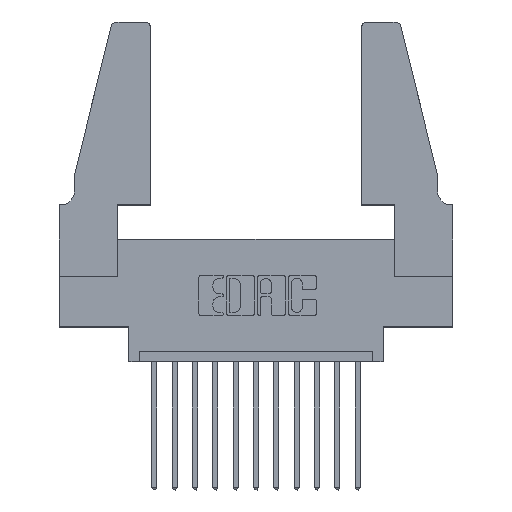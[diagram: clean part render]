
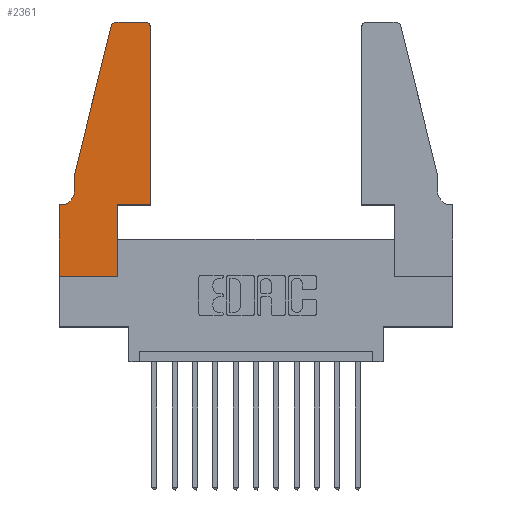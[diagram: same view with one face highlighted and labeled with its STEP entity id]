
A CAD part, top view. The second image highlights one B-rep face of the part: STEP entity #2361.
In plain terms, the highlighted planar face has unit normal (0, 0, 1).
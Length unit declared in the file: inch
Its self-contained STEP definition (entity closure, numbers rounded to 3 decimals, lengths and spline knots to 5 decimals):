
#89 = CARTESIAN_POINT ( 'NONE',  ( 0.4505, 0.35, 0.37 ) ) ;
#116 = CARTESIAN_POINT ( 'NONE',  ( 0.25487, 1.22718, 0.37 ) ) ;
#725 = CARTESIAN_POINT ( 'NONE',  ( 0.4505, 0.35, 0.37 ) ) ;
#737 = EDGE_CURVE ( 'NONE', #4386, #1891, #3913, .T. ) ;
#766 = LINE ( 'NONE', #13095, #12491 ) ;
#920 = EDGE_CURVE ( 'NONE', #3782, #13188, #6446, .T. ) ;
#1438 = DIRECTION ( 'NONE',  ( 0., 0., 1. ) ) ;
#1468 = DIRECTION ( 'NONE',  ( 1., 0., 0. ) ) ;
#1543 = VECTOR ( 'NONE', #6081, 39.37008 ) ;
#1684 = DIRECTION ( 'NONE',  ( 0., -1., 0. ) ) ;
#1845 = EDGE_CURVE ( 'NONE', #1891, #2045, #13556, .T. ) ;
#1891 = VERTEX_POINT ( 'NONE', #8064 ) ;
#2045 = VERTEX_POINT ( 'NONE', #2785 ) ;
#2224 = LINE ( 'NONE', #14185, #1543 ) ;
#2236 = VERTEX_POINT ( 'NONE', #14622 ) ;
#2361 = ADVANCED_FACE ( 'NONE', ( #10120 ), #10490, .T. ) ;
#2376 = EDGE_CURVE ( 'NONE', #3170, #7698, #11215, .T. ) ;
#2407 = ORIENTED_EDGE ( 'NONE', *, *, #13330, .T. ) ;
#2785 = CARTESIAN_POINT ( 'NONE',  ( 0., 0.35, 0.37 ) ) ;
#2909 = DIRECTION ( 'NONE',  ( 0., 1., 0. ) ) ;
#2993 = LINE ( 'NONE', #14517, #6554 ) ;
#3170 = VERTEX_POINT ( 'NONE', #116 ) ;
#3244 = LINE ( 'NONE', #6177, #12352 ) ;
#3681 = DIRECTION ( 'NONE',  ( 1., 0., 0. ) ) ;
#3738 = ORIENTED_EDGE ( 'NONE', *, *, #2376, .T. ) ;
#3782 = VERTEX_POINT ( 'NONE', #89 ) ;
#3790 = CARTESIAN_POINT ( 'NONE',  ( 0.0755, 0.5, 0.37 ) ) ;
#3913 = CIRCLE ( 'NONE', #10868, 0.07 ) ;
#4011 = CARTESIAN_POINT ( 'NONE',  ( 0.2865, 0.35, 0.37 ) ) ;
#4113 = ORIENTED_EDGE ( 'NONE', *, *, #9450, .T. ) ;
#4261 = DIRECTION ( 'NONE',  ( 0., 1., 0. ) ) ;
#4386 = VERTEX_POINT ( 'NONE', #6776 ) ;
#4493 = CARTESIAN_POINT ( 'NONE',  ( 0.0055, 0.42, 0.37 ) ) ;
#4815 = DIRECTION ( 'NONE',  ( -0.239, -0.971, 0. ) ) ;
#4913 = CIRCLE ( 'NONE', #4923, 0.03 ) ;
#4922 = DIRECTION ( 'NONE',  ( 0., 0., 1. ) ) ;
#4923 = AXIS2_PLACEMENT_3D ( 'NONE', #12338, #12143, #13402 ) ;
#4983 = VECTOR ( 'NONE', #12726, 39.37008 ) ;
#5013 = CARTESIAN_POINT ( 'NONE',  ( 0.0755, 0.5, 0.37 ) ) ;
#5110 = ORIENTED_EDGE ( 'NONE', *, *, #11176, .T. ) ;
#5371 = VERTEX_POINT ( 'NONE', #7782 ) ;
#5526 = AXIS2_PLACEMENT_3D ( 'NONE', #9406, #4922, #1468 ) ;
#5924 = ORIENTED_EDGE ( 'NONE', *, *, #8864, .T. ) ;
#6081 = DIRECTION ( 'NONE',  ( 1., 0., 0. ) ) ;
#6177 = CARTESIAN_POINT ( 'NONE',  ( 0.2605, 1.25, 0.37 ) ) ;
#6446 = LINE ( 'NONE', #725, #7123 ) ;
#6554 = VECTOR ( 'NONE', #4261, 39.37008 ) ;
#6776 = CARTESIAN_POINT ( 'NONE',  ( 0.0755, 0.42, 0.37 ) ) ;
#7045 = VERTEX_POINT ( 'NONE', #13033 ) ;
#7113 = LINE ( 'NONE', #11530, #4983 ) ;
#7123 = VECTOR ( 'NONE', #2909, 39.37008 ) ;
#7177 = VECTOR ( 'NONE', #11707, 39.37008 ) ;
#7354 = EDGE_CURVE ( 'NONE', #14381, #14234, #2993, .T. ) ;
#7688 = CIRCLE ( 'NONE', #11392, 0.03 ) ;
#7698 = VERTEX_POINT ( 'NONE', #3790 ) ;
#7782 = CARTESIAN_POINT ( 'NONE',  ( 0., 0., 0.37 ) ) ;
#8064 = CARTESIAN_POINT ( 'NONE',  ( 0.0055, 0.35, 0.37 ) ) ;
#8535 = VECTOR ( 'NONE', #9864, 39.37008 ) ;
#8864 = EDGE_CURVE ( 'NONE', #7698, #4386, #12046, .T. ) ;
#8868 = ORIENTED_EDGE ( 'NONE', *, *, #737, .T. ) ;
#8895 = ORIENTED_EDGE ( 'NONE', *, *, #7354, .T. ) ;
#9120 = DIRECTION ( 'NONE',  ( -1., 0., 0. ) ) ;
#9406 = CARTESIAN_POINT ( 'NONE',  ( 0., 0.35, 0.37 ) ) ;
#9450 = EDGE_CURVE ( 'NONE', #7045, #3170, #7688, .T. ) ;
#9759 = DIRECTION ( 'NONE',  ( -1., 0., 0. ) ) ;
#9864 = DIRECTION ( 'NONE',  ( -1., 0., 0. ) ) ;
#10120 = FACE_OUTER_BOUND ( 'NONE', #14323, .T. ) ;
#10127 = ORIENTED_EDGE ( 'NONE', *, *, #920, .T. ) ;
#10253 = EDGE_CURVE ( 'NONE', #2236, #7045, #3244, .T. ) ;
#10368 = CARTESIAN_POINT ( 'NONE',  ( 0.284, 1.22, 0.37 ) ) ;
#10490 = PLANE ( 'NONE',  #5526 ) ;
#10868 = AXIS2_PLACEMENT_3D ( 'NONE', #4493, #13784, #9120 ) ;
#10938 = ORIENTED_EDGE ( 'NONE', *, *, #1845, .T. ) ;
#11005 = ORIENTED_EDGE ( 'NONE', *, *, #10253, .T. ) ;
#11176 = EDGE_CURVE ( 'NONE', #5371, #14381, #7113, .T. ) ;
#11215 = LINE ( 'NONE', #11669, #11940 ) ;
#11320 = EDGE_CURVE ( 'NONE', #2045, #5371, #766, .T. ) ;
#11392 = AXIS2_PLACEMENT_3D ( 'NONE', #10368, #1438, #3681 ) ;
#11530 = CARTESIAN_POINT ( 'NONE',  ( 0., 0., 0.37 ) ) ;
#11666 = ORIENTED_EDGE ( 'NONE', *, *, #12839, .T. ) ;
#11669 = CARTESIAN_POINT ( 'NONE',  ( 0.0755, 0.5, 0.37 ) ) ;
#11707 = DIRECTION ( 'NONE',  ( 0., -1., 0. ) ) ;
#11940 = VECTOR ( 'NONE', #4815, 39.37008 ) ;
#12046 = LINE ( 'NONE', #5013, #7177 ) ;
#12143 = DIRECTION ( 'NONE',  ( 0., 0., 1. ) ) ;
#12338 = CARTESIAN_POINT ( 'NONE',  ( 0.4205, 1.22, 0.37 ) ) ;
#12352 = VECTOR ( 'NONE', #9759, 39.37008 ) ;
#12491 = VECTOR ( 'NONE', #1684, 39.37008 ) ;
#12726 = DIRECTION ( 'NONE',  ( 1., 0., 0. ) ) ;
#12839 = EDGE_CURVE ( 'NONE', #13188, #2236, #4913, .T. ) ;
#13033 = CARTESIAN_POINT ( 'NONE',  ( 0.284, 1.25, 0.37 ) ) ;
#13095 = CARTESIAN_POINT ( 'NONE',  ( 0., 0., 0.37 ) ) ;
#13188 = VERTEX_POINT ( 'NONE', #13726 ) ;
#13330 = EDGE_CURVE ( 'NONE', #14234, #3782, #2224, .T. ) ;
#13402 = DIRECTION ( 'NONE',  ( 1., 0., 0. ) ) ;
#13415 = ORIENTED_EDGE ( 'NONE', *, *, #11320, .T. ) ;
#13556 = LINE ( 'NONE', #14422, #8535 ) ;
#13726 = CARTESIAN_POINT ( 'NONE',  ( 0.4505, 1.22, 0.37 ) ) ;
#13784 = DIRECTION ( 'NONE',  ( 0., 0., -1. ) ) ;
#14185 = CARTESIAN_POINT ( 'NONE',  ( 0.4505, 0.35, 0.37 ) ) ;
#14234 = VERTEX_POINT ( 'NONE', #4011 ) ;
#14323 = EDGE_LOOP ( 'NONE', ( #11005, #4113, #3738, #5924, #8868, #10938, #13415, #5110, #8895, #2407, #10127, #11666 ) ) ;
#14381 = VERTEX_POINT ( 'NONE', #14458 ) ;
#14422 = CARTESIAN_POINT ( 'NONE',  ( 0.0755, 0.35, 0.37 ) ) ;
#14458 = CARTESIAN_POINT ( 'NONE',  ( 0.2865, 0., 0.37 ) ) ;
#14517 = CARTESIAN_POINT ( 'NONE',  ( 0.2865, 0.35, 0.37 ) ) ;
#14622 = CARTESIAN_POINT ( 'NONE',  ( 0.4205, 1.25, 0.37 ) ) ;
